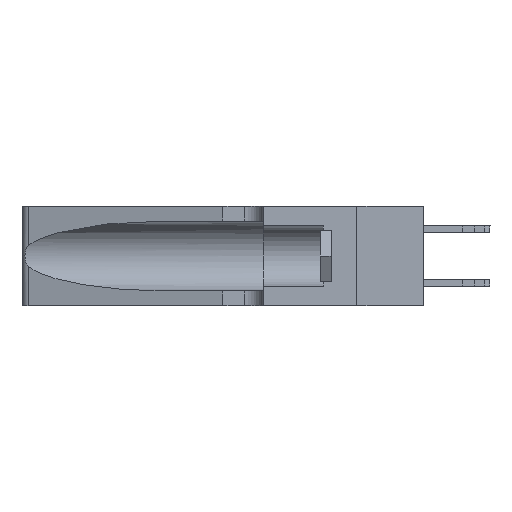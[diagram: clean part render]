
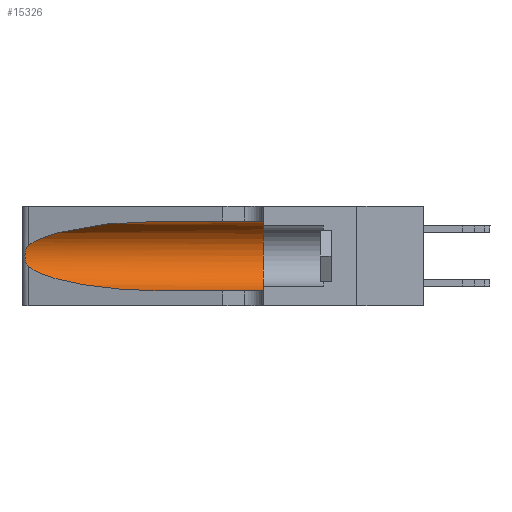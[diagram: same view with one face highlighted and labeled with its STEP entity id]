
A CAD part, left-side view. The second image highlights one B-rep face of the part: STEP entity #15326.
In plain terms, the highlighted cylindrical face has radius 3.308 mm (diameter 6.617 mm), a partial arc.
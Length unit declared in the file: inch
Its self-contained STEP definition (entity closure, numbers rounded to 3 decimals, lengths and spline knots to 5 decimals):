
#698 = CARTESIAN_POINT ( 'NONE',  ( 0.25639, 1.23186, 0.15144 ) ) ;
#1309 = LINE ( 'NONE', #19076, #25327 ) ;
#1321 = DIRECTION ( 'NONE',  ( 0., -1., 0. ) ) ;
#1575 = CARTESIAN_POINT ( 'NONE',  ( 0.25487, 1.22718, 0.22369 ) ) ;
#1887 = VERTEX_POINT ( 'NONE', #28360 ) ;
#1969 = DIRECTION ( 'NONE',  ( 0., 0., -1. ) ) ;
#2817 = EDGE_CURVE ( 'NONE', #14312, #3367, #4768, .T. ) ;
#2837 = ORIENTED_EDGE ( 'NONE', *, *, #17386, .T. ) ;
#3367 = VERTEX_POINT ( 'NONE', #26879 ) ;
#3462 = CARTESIAN_POINT ( 'NONE',  ( 0.25487, 1.22718, 0.14631 ) ) ;
#3480 = CARTESIAN_POINT ( 'NONE',  ( 0.1305, 0.72297, 0.31525 ) ) ;
#3580 = CARTESIAN_POINT ( 'NONE',  ( 0.25487, 1.22718, 0.22369 ) ) ;
#4243 = ORIENTED_EDGE ( 'NONE', *, *, #10148, .F. ) ;
#4642 = VERTEX_POINT ( 'NONE', #18004 ) ;
#4768 = LINE ( 'NONE', #23561, #26358 ) ;
#5576 = CARTESIAN_POINT ( 'NONE',  ( 0.1305, 0.35, 0.185 ) ) ;
#5819 = CARTESIAN_POINT ( 'NONE',  ( 0.1305, 0.72297, 0.31525 ) ) ;
#6082 = VERTEX_POINT ( 'NONE', #13908 ) ;
#6243 = CARTESIAN_POINT ( 'NONE',  ( 0.25787, 1.23484, 0.2124 ) ) ;
#7377 = CARTESIAN_POINT ( 'NONE',  ( 0.25555, 1.22993, 0.14849 ) ) ;
#7723 = DIRECTION ( 'NONE',  ( 0., -1., 0. ) ) ;
#8242 = CARTESIAN_POINT ( 'NONE',  ( 0.18966, 0.96281, 0.05475 ) ) ;
#8425 = ORIENTED_EDGE ( 'NONE', *, *, #25299, .T. ) ;
#8500 = CARTESIAN_POINT ( 'NONE',  ( 0.25854, 1.2359, 0.20912 ) ) ;
#8664 = CARTESIAN_POINT ( 'NONE',  ( 0.25639, 1.23184, 0.21858 ) ) ;
#8688 = CARTESIAN_POINT ( 'NONE',  ( 0.1305, 0.35, 0.05475 ) ) ;
#8691 = CARTESIAN_POINT ( 'NONE',  ( 0.26075, 1.23896, 0.178 ) ) ;
#8975 = CARTESIAN_POINT ( 'NONE',  ( 0.26017, 1.23833, 0.17102 ) ) ;
#9749 = CARTESIAN_POINT ( 'NONE',  ( 0.25487, 1.22718, 0.14631 ) ) ;
#9994 =( BOUNDED_CURVE ( )  B_SPLINE_CURVE ( 3, ( #3480, #14904, #21656, #3580 ),
 .UNSPECIFIED., .F., .F. ) 
 B_SPLINE_CURVE_WITH_KNOTS ( ( 4, 4 ),
 ( 1.5708, 2.84003 ),
 .UNSPECIFIED. ) 
 CURVE ( )  GEOMETRIC_REPRESENTATION_ITEM ( )  RATIONAL_B_SPLINE_CURVE ( ( 1., 0.87, 0.87, 1. ) ) 
 REPRESENTATION_ITEM ( '' )  );
#10037 = DIRECTION ( 'NONE',  ( 0., -1., 0. ) ) ;
#10148 = EDGE_CURVE ( 'NONE', #3367, #14570, #26854, .T. ) ;
#10309 = ORIENTED_EDGE ( 'NONE', *, *, #12907, .T. ) ;
#11218 = AXIS2_PLACEMENT_3D ( 'NONE', #28208, #10037, #1969 ) ;
#12186 = DIRECTION ( 'NONE',  ( 0., 0., 1. ) ) ;
#12907 = EDGE_CURVE ( 'NONE', #4642, #6082, #26977, .T. ) ;
#12972 = CARTESIAN_POINT ( 'NONE',  ( 0.2373, 1.15595, 0.08982 ) ) ;
#13908 = CARTESIAN_POINT ( 'NONE',  ( 0.25487, 1.22718, 0.14631 ) ) ;
#14177 = DIRECTION ( 'NONE',  ( 0., 1., 0. ) ) ;
#14312 = VERTEX_POINT ( 'NONE', #5819 ) ;
#14570 = VERTEX_POINT ( 'NONE', #8688 ) ;
#14904 = CARTESIAN_POINT ( 'NONE',  ( 0.18966, 0.96281, 0.31525 ) ) ;
#14947 = CYLINDRICAL_SURFACE ( 'NONE', #11218, 0.13025 ) ;
#15326 = ADVANCED_FACE ( 'NONE', ( #22300 ), #14947, .F. ) ;
#15340 = CARTESIAN_POINT ( 'NONE',  ( 0.26075, 1.23896, 0.19203 ) ) ;
#17386 = EDGE_CURVE ( 'NONE', #1887, #14570, #1309, .T. ) ;
#18004 = CARTESIAN_POINT ( 'NONE',  ( 0.25487, 1.22718, 0.22369 ) ) ;
#19076 = CARTESIAN_POINT ( 'NONE',  ( 0.1305, 1.61858, 0.05475 ) ) ;
#20289 = CARTESIAN_POINT ( 'NONE',  ( 0.25856, 1.23593, 0.16098 ) ) ;
#20458 =( BOUNDED_CURVE ( )  B_SPLINE_CURVE ( 3, ( #3462, #12972, #8242, #26274 ),
 .UNSPECIFIED., .F., .T. ) 
 B_SPLINE_CURVE_WITH_KNOTS ( ( 4, 4 ),
 ( 3.44316, 4.71239 ),
 .UNSPECIFIED. ) 
 CURVE ( )  GEOMETRIC_REPRESENTATION_ITEM ( )  RATIONAL_B_SPLINE_CURVE ( ( 1., 0.87, 0.87, 1. ) ) 
 REPRESENTATION_ITEM ( '' )  );
#20879 = CARTESIAN_POINT ( 'NONE',  ( 0.25789, 1.23486, 0.15765 ) ) ;
#20968 = ORIENTED_EDGE ( 'NONE', *, *, #26076, .T. ) ;
#21656 = CARTESIAN_POINT ( 'NONE',  ( 0.2373, 1.15595, 0.28018 ) ) ;
#22161 = CARTESIAN_POINT ( 'NONE',  ( 0.25555, 1.22994, 0.2215 ) ) ;
#22300 = FACE_OUTER_BOUND ( 'NONE', #27034, .T. ) ;
#23561 = CARTESIAN_POINT ( 'NONE',  ( 0.1305, 1.61858, 0.31525 ) ) ;
#24871 = ORIENTED_EDGE ( 'NONE', *, *, #2817, .F. ) ;
#25299 = EDGE_CURVE ( 'NONE', #6082, #1887, #20458, .T. ) ;
#25327 = VECTOR ( 'NONE', #1321, 39.37008 ) ;
#26076 = EDGE_CURVE ( 'NONE', #14312, #4642, #9994, .T. ) ;
#26274 = CARTESIAN_POINT ( 'NONE',  ( 0.1305, 0.72297, 0.05475 ) ) ;
#26358 = VECTOR ( 'NONE', #7723, 39.37008 ) ;
#26854 = CIRCLE ( 'NONE', #28828, 0.13025 ) ;
#26879 = CARTESIAN_POINT ( 'NONE',  ( 0.1305, 0.35, 0.31525 ) ) ;
#26977 = B_SPLINE_CURVE_WITH_KNOTS ( 'NONE', 3,
 ( #1575, #22161, #8664, #6243, #8500, #28748, #15340, #8691, #8975, #20289, #20879, #698, #7377, #9749 ),
 .UNSPECIFIED., .F., .F.,
 ( 4, 2, 2, 2, 2, 2, 4 ),
 ( 0., 0.00027, 0.00053, 0.00107, 0.0016, 0.00187, 0.00214 ),
 .UNSPECIFIED. ) ;
#27034 = EDGE_LOOP ( 'NONE', ( #20968, #10309, #8425, #2837, #4243, #24871 ) ) ;
#28208 = CARTESIAN_POINT ( 'NONE',  ( 0.1305, 1.61858, 0.185 ) ) ;
#28360 = CARTESIAN_POINT ( 'NONE',  ( 0.1305, 0.72297, 0.05475 ) ) ;
#28748 = CARTESIAN_POINT ( 'NONE',  ( 0.26018, 1.23835, 0.19895 ) ) ;
#28828 = AXIS2_PLACEMENT_3D ( 'NONE', #5576, #14177, #12186 ) ;
